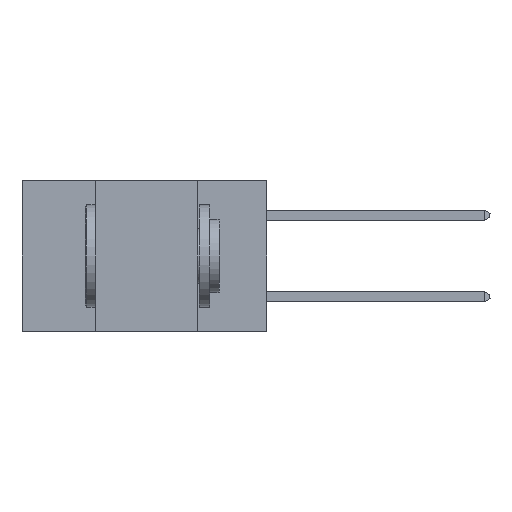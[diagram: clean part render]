
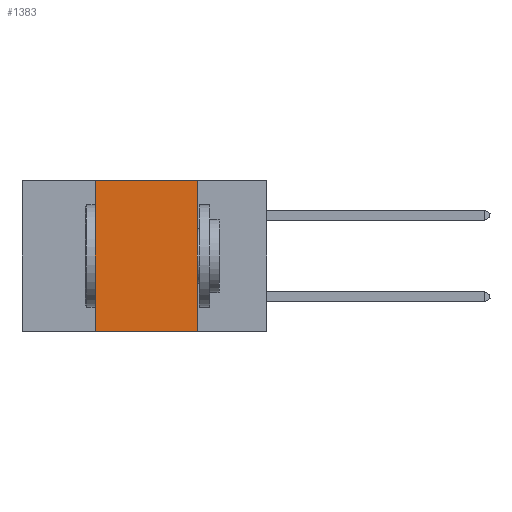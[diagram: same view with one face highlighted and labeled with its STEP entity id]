
A CAD part, left-side view. The second image highlights one B-rep face of the part: STEP entity #1383.
In plain terms, the highlighted planar face has unit normal (-1, 0, 0).
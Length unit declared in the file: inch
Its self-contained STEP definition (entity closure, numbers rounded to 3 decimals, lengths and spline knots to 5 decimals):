
#1383 = ADVANCED_FACE ( 'NONE', ( #24827 ), #6246, .F. ) ;
#1669 = EDGE_CURVE ( 'NONE', #32531, #7141, #7963, .T. ) ;
#2172 = CARTESIAN_POINT ( 'NONE',  ( 0., 0.42, -0.37 ) ) ;
#4722 = DIRECTION ( 'NONE',  ( 0., -1., 0. ) ) ;
#5237 = AXIS2_PLACEMENT_3D ( 'NONE', #25058, #15926, #6107 ) ;
#6107 = DIRECTION ( 'NONE',  ( 0., 0., -1. ) ) ;
#6246 = PLANE ( 'NONE',  #5237 ) ;
#6713 = VERTEX_POINT ( 'NONE', #8421 ) ;
#7141 = VERTEX_POINT ( 'NONE', #11516 ) ;
#7963 = LINE ( 'NONE', #10806, #36690 ) ;
#8421 = CARTESIAN_POINT ( 'NONE',  ( 0., 0.17, 0. ) ) ;
#10806 = CARTESIAN_POINT ( 'NONE',  ( 0., 0.6, -0.37 ) ) ;
#11325 = LINE ( 'NONE', #33615, #15279 ) ;
#11516 = CARTESIAN_POINT ( 'NONE',  ( 0., 0.17, -0.37 ) ) ;
#12203 = EDGE_CURVE ( 'NONE', #6713, #7141, #16420, .T. ) ;
#13396 = ORIENTED_EDGE ( 'NONE', *, *, #33591, .F. ) ;
#14437 = VECTOR ( 'NONE', #17346, 39.37008 ) ;
#15279 = VECTOR ( 'NONE', #17858, 39.37008 ) ;
#15926 = DIRECTION ( 'NONE',  ( 1., 0., 0. ) ) ;
#16420 = LINE ( 'NONE', #29644, #14437 ) ;
#17326 = CARTESIAN_POINT ( 'NONE',  ( 0., 0.6, 0. ) ) ;
#17346 = DIRECTION ( 'NONE',  ( 0., 0., -1. ) ) ;
#17858 = DIRECTION ( 'NONE',  ( 0., 0., 1. ) ) ;
#18456 = ORIENTED_EDGE ( 'NONE', *, *, #12203, .F. ) ;
#19467 = CARTESIAN_POINT ( 'NONE',  ( 0., 0.42, 0. ) ) ;
#19798 = LINE ( 'NONE', #17326, #26696 ) ;
#20531 = ORIENTED_EDGE ( 'NONE', *, *, #1669, .T. ) ;
#24827 = FACE_OUTER_BOUND ( 'NONE', #33717, .T. ) ;
#25058 = CARTESIAN_POINT ( 'NONE',  ( 0., 0.6, 0. ) ) ;
#25088 = EDGE_CURVE ( 'NONE', #37344, #6713, #19798, .T. ) ;
#26696 = VECTOR ( 'NONE', #33503, 39.37008 ) ;
#29644 = CARTESIAN_POINT ( 'NONE',  ( 0., 0.17, 0. ) ) ;
#32531 = VERTEX_POINT ( 'NONE', #2172 ) ;
#33503 = DIRECTION ( 'NONE',  ( 0., -1., 0. ) ) ;
#33591 = EDGE_CURVE ( 'NONE', #32531, #37344, #11325, .T. ) ;
#33615 = CARTESIAN_POINT ( 'NONE',  ( 0., 0.42, 0. ) ) ;
#33717 = EDGE_LOOP ( 'NONE', ( #18456, #40401, #13396, #20531 ) ) ;
#36690 = VECTOR ( 'NONE', #4722, 39.37008 ) ;
#37344 = VERTEX_POINT ( 'NONE', #19467 ) ;
#40401 = ORIENTED_EDGE ( 'NONE', *, *, #25088, .F. ) ;
